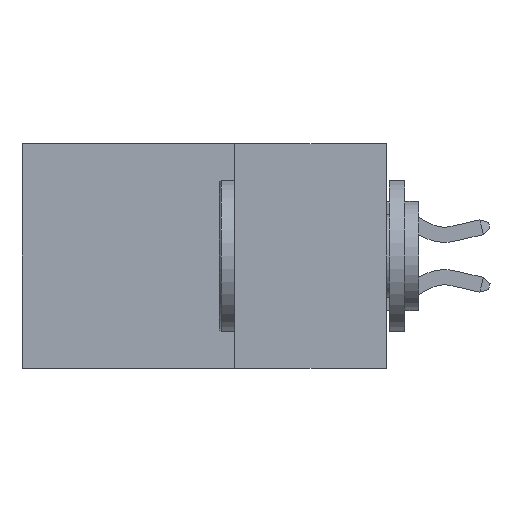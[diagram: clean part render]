
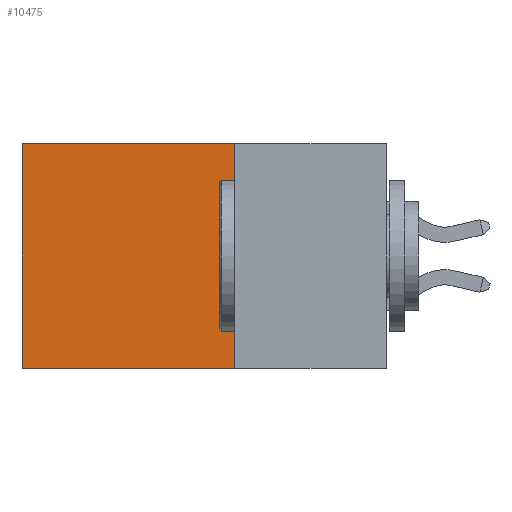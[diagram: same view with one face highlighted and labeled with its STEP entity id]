
A CAD part, left-side view. The second image highlights one B-rep face of the part: STEP entity #10475.
In plain terms, the highlighted planar face has unit normal (-1, 0, 0).
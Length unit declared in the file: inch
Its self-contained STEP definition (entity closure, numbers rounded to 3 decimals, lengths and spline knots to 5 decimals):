
#276 = CARTESIAN_POINT ( 'NONE',  ( 0.298, 0.25, 0. ) ) ;
#332 = EDGE_CURVE ( 'NONE', #3588, #2745, #2113, .T. ) ;
#460 = CARTESIAN_POINT ( 'NONE',  ( 0.298, 0.25, 0. ) ) ;
#825 = CARTESIAN_POINT ( 'NONE',  ( 0.298, 0.25, -0.37 ) ) ;
#1608 = DIRECTION ( 'NONE',  ( 0., 0., -1. ) ) ;
#2074 = EDGE_CURVE ( 'NONE', #2745, #3252, #9289, .T. ) ;
#2113 = LINE ( 'NONE', #276, #11812 ) ;
#2238 = ORIENTED_EDGE ( 'NONE', *, *, #4314, .F. ) ;
#2340 = ORIENTED_EDGE ( 'NONE', *, *, #8997, .F. ) ;
#2505 = CARTESIAN_POINT ( 'NONE',  ( 0.298, 0.25, -0.37 ) ) ;
#2745 = VERTEX_POINT ( 'NONE', #7699 ) ;
#2849 = CARTESIAN_POINT ( 'NONE',  ( 0.298, 0.6, 0. ) ) ;
#3252 = VERTEX_POINT ( 'NONE', #9411 ) ;
#3556 = CARTESIAN_POINT ( 'NONE',  ( 0.298, 0.25, 0. ) ) ;
#3588 = VERTEX_POINT ( 'NONE', #460 ) ;
#3659 = LINE ( 'NONE', #9249, #4849 ) ;
#4228 = FACE_OUTER_BOUND ( 'NONE', #10829, .T. ) ;
#4314 = EDGE_CURVE ( 'NONE', #7268, #3252, #5409, .T. ) ;
#4849 = VECTOR ( 'NONE', #1608, 39.37008 ) ;
#5409 = LINE ( 'NONE', #2505, #10988 ) ;
#6420 = DIRECTION ( 'NONE',  ( 0., 0., -1. ) ) ;
#6898 = DIRECTION ( 'NONE',  ( 0., 1., 0. ) ) ;
#7268 = VERTEX_POINT ( 'NONE', #825 ) ;
#7386 = VECTOR ( 'NONE', #10870, 39.37008 ) ;
#7699 = CARTESIAN_POINT ( 'NONE',  ( 0.298, 0.6, 0. ) ) ;
#8006 = ORIENTED_EDGE ( 'NONE', *, *, #332, .T. ) ;
#8997 = EDGE_CURVE ( 'NONE', #3588, #7268, #3659, .T. ) ;
#9249 = CARTESIAN_POINT ( 'NONE',  ( 0.298, 0.25, 0. ) ) ;
#9289 = LINE ( 'NONE', #2849, #7386 ) ;
#9411 = CARTESIAN_POINT ( 'NONE',  ( 0.298, 0.6, -0.37 ) ) ;
#10131 = DIRECTION ( 'NONE',  ( 1., 0., 0. ) ) ;
#10475 = ADVANCED_FACE ( 'NONE', ( #4228 ), #12059, .F. ) ;
#10743 = ORIENTED_EDGE ( 'NONE', *, *, #2074, .T. ) ;
#10829 = EDGE_LOOP ( 'NONE', ( #10743, #2238, #2340, #8006 ) ) ;
#10870 = DIRECTION ( 'NONE',  ( 0., 0., -1. ) ) ;
#10988 = VECTOR ( 'NONE', #11838, 39.37008 ) ;
#11386 = AXIS2_PLACEMENT_3D ( 'NONE', #3556, #10131, #6420 ) ;
#11812 = VECTOR ( 'NONE', #6898, 39.37008 ) ;
#11838 = DIRECTION ( 'NONE',  ( 0., 1., 0. ) ) ;
#12059 = PLANE ( 'NONE',  #11386 ) ;
